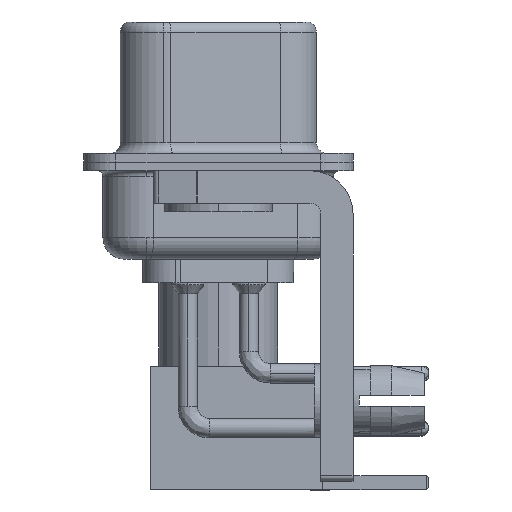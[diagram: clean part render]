
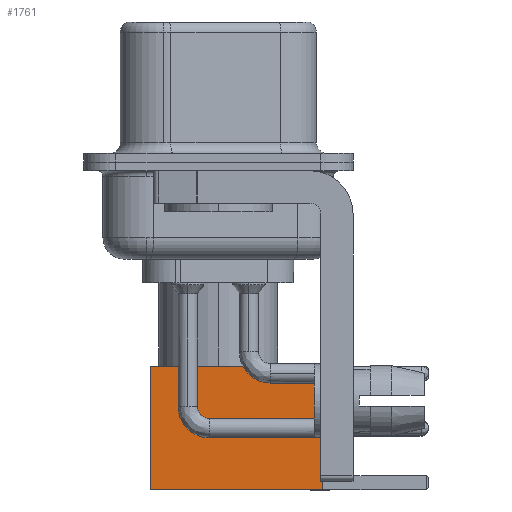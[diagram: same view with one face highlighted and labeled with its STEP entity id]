
A CAD part, left-side view. The second image highlights one B-rep face of the part: STEP entity #1761.
In plain terms, the highlighted face is planar.
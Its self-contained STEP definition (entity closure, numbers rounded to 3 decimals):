
#36 = CARTESIAN_POINT ( 'NONE',  ( 0., 2.875, 8. ) ) ;
#170 = CARTESIAN_POINT ( 'NONE',  ( -2.875, 2.875, 0. ) ) ;
#371 = PLANE ( 'NONE',  #15227 ) ;
#1244 = VERTEX_POINT ( 'NONE', #10255 ) ;
#1761 = ADVANCED_FACE ( 'NONE', ( #4526 ), #371, .T. ) ;
#3504 = ORIENTED_EDGE ( 'NONE', *, *, #6143, .F. ) ;
#4059 = LINE ( 'NONE', #36, #17985 ) ;
#4526 = FACE_OUTER_BOUND ( 'NONE', #16419, .T. ) ;
#6143 = EDGE_CURVE ( 'NONE', #22944, #21261, #20061, .T. ) ;
#6213 = DIRECTION ( 'NONE',  ( 0., 0., 1. ) ) ;
#6306 = ORIENTED_EDGE ( 'NONE', *, *, #25042, .F. ) ;
#8285 = CARTESIAN_POINT ( 'NONE',  ( 2.875, 2.875, 0. ) ) ;
#9014 = DIRECTION ( 'NONE',  ( 0., 0., -1. ) ) ;
#10047 = CARTESIAN_POINT ( 'NONE',  ( 0., 2.875, 0. ) ) ;
#10255 = CARTESIAN_POINT ( 'NONE',  ( 2.875, 2.875, 0. ) ) ;
#10689 = EDGE_CURVE ( 'NONE', #1244, #21261, #13833, .T. ) ;
#10713 = CARTESIAN_POINT ( 'NONE',  ( 2.875, 2.875, 0. ) ) ;
#11737 = DIRECTION ( 'NONE',  ( -1., 0., 0. ) ) ;
#12579 = DIRECTION ( 'NONE',  ( 0., 1., 0. ) ) ;
#12637 = DIRECTION ( 'NONE',  ( 0., 0., -1. ) ) ;
#13049 = LINE ( 'NONE', #10713, #21709 ) ;
#13833 = LINE ( 'NONE', #10047, #19029 ) ;
#15096 = CARTESIAN_POINT ( 'NONE',  ( -2.875, 2.875, 8. ) ) ;
#15227 = AXIS2_PLACEMENT_3D ( 'NONE', #8285, #12579, #6213 ) ;
#15253 = CARTESIAN_POINT ( 'NONE',  ( 2.875, 2.875, 8. ) ) ;
#16419 = EDGE_LOOP ( 'NONE', ( #19218, #16688, #3504, #6306 ) ) ;
#16688 = ORIENTED_EDGE ( 'NONE', *, *, #10689, .T. ) ;
#17985 = VECTOR ( 'NONE', #21880, 1000. ) ;
#18480 = CARTESIAN_POINT ( 'NONE',  ( -2.875, 2.875, 0. ) ) ;
#19029 = VECTOR ( 'NONE', #11737, 1000. ) ;
#19218 = ORIENTED_EDGE ( 'NONE', *, *, #24246, .T. ) ;
#19731 = VECTOR ( 'NONE', #12637, 1000. ) ;
#20061 = LINE ( 'NONE', #170, #19731 ) ;
#21261 = VERTEX_POINT ( 'NONE', #18480 ) ;
#21709 = VECTOR ( 'NONE', #9014, 1000. ) ;
#21880 = DIRECTION ( 'NONE',  ( -1., 0., 0. ) ) ;
#22449 = VERTEX_POINT ( 'NONE', #15253 ) ;
#22944 = VERTEX_POINT ( 'NONE', #15096 ) ;
#24246 = EDGE_CURVE ( 'NONE', #22449, #1244, #13049, .T. ) ;
#25042 = EDGE_CURVE ( 'NONE', #22449, #22944, #4059, .T. ) ;
